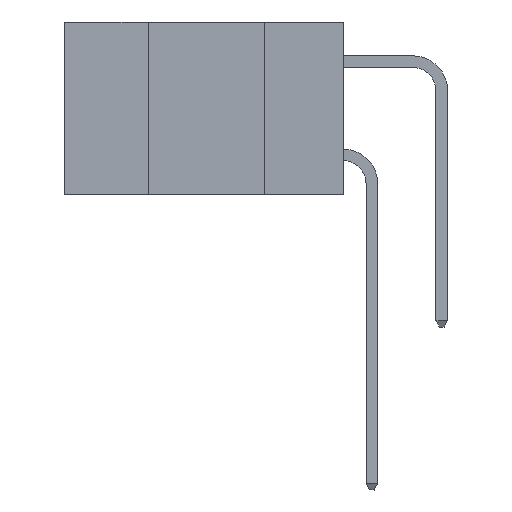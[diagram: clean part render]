
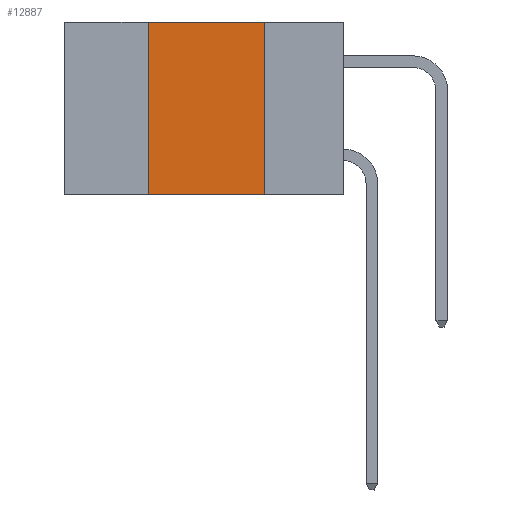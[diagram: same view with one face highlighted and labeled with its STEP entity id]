
A CAD part, left-side view. The second image highlights one B-rep face of the part: STEP entity #12887.
In plain terms, the highlighted planar face has unit normal (-1, 0, 0).
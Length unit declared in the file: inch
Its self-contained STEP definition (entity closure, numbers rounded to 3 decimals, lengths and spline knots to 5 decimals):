
#407 = LINE ( 'NONE', #10537, #13648 ) ;
#583 = DIRECTION ( 'NONE',  ( 0., -1., 0. ) ) ;
#591 = DIRECTION ( 'NONE',  ( 0., 0., -1. ) ) ;
#2275 = VERTEX_POINT ( 'NONE', #6621 ) ;
#2342 = ORIENTED_EDGE ( 'NONE', *, *, #10700, .F. ) ;
#2628 = DIRECTION ( 'NONE',  ( 1., 0., 0. ) ) ;
#2801 = LINE ( 'NONE', #8890, #14022 ) ;
#3231 = CARTESIAN_POINT ( 'NONE',  ( 0., 0.17, 0. ) ) ;
#3431 = LINE ( 'NONE', #8037, #14328 ) ;
#3582 = AXIS2_PLACEMENT_3D ( 'NONE', #16279, #2628, #17474 ) ;
#3915 = PLANE ( 'NONE',  #3582 ) ;
#4095 = FACE_OUTER_BOUND ( 'NONE', #7981, .T. ) ;
#6358 = EDGE_CURVE ( 'NONE', #2275, #12626, #13322, .T. ) ;
#6484 = ORIENTED_EDGE ( 'NONE', *, *, #6358, .T. ) ;
#6505 = ORIENTED_EDGE ( 'NONE', *, *, #14348, .F. ) ;
#6621 = CARTESIAN_POINT ( 'NONE',  ( 0., 0.42, -0.37 ) ) ;
#7981 = EDGE_LOOP ( 'NONE', ( #6505, #18867, #2342, #6484 ) ) ;
#8037 = CARTESIAN_POINT ( 'NONE',  ( 0., 0.6, 0. ) ) ;
#8793 = DIRECTION ( 'NONE',  ( 0., 0., 1. ) ) ;
#8890 = CARTESIAN_POINT ( 'NONE',  ( 0., 0.42, -0.37 ) ) ;
#8996 = CARTESIAN_POINT ( 'NONE',  ( 0., 0.42, 0. ) ) ;
#10537 = CARTESIAN_POINT ( 'NONE',  ( 0., 0.17, -0.37 ) ) ;
#10700 = EDGE_CURVE ( 'NONE', #2275, #16934, #2801, .T. ) ;
#12626 = VERTEX_POINT ( 'NONE', #16357 ) ;
#12887 = ADVANCED_FACE ( 'NONE', ( #4095 ), #3915, .F. ) ;
#13322 = LINE ( 'NONE', #19434, #18682 ) ;
#13648 = VECTOR ( 'NONE', #591, 39.37008 ) ;
#14022 = VECTOR ( 'NONE', #8793, 39.37008 ) ;
#14328 = VECTOR ( 'NONE', #15805, 39.37008 ) ;
#14348 = EDGE_CURVE ( 'NONE', #16619, #12626, #407, .T. ) ;
#15805 = DIRECTION ( 'NONE',  ( 0., -1., 0. ) ) ;
#16279 = CARTESIAN_POINT ( 'NONE',  ( 0., 0.6, 0. ) ) ;
#16357 = CARTESIAN_POINT ( 'NONE',  ( 0., 0.17, -0.37 ) ) ;
#16619 = VERTEX_POINT ( 'NONE', #3231 ) ;
#16934 = VERTEX_POINT ( 'NONE', #8996 ) ;
#17474 = DIRECTION ( 'NONE',  ( 0., 0., -1. ) ) ;
#18230 = EDGE_CURVE ( 'NONE', #16934, #16619, #3431, .T. ) ;
#18682 = VECTOR ( 'NONE', #583, 39.37008 ) ;
#18867 = ORIENTED_EDGE ( 'NONE', *, *, #18230, .F. ) ;
#19434 = CARTESIAN_POINT ( 'NONE',  ( 0., 0.6, -0.37 ) ) ;
